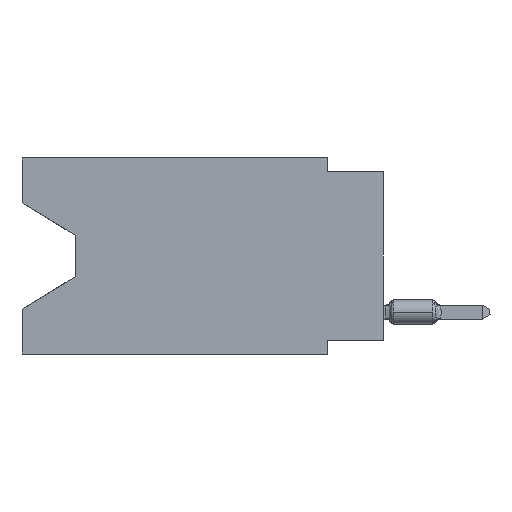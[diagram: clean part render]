
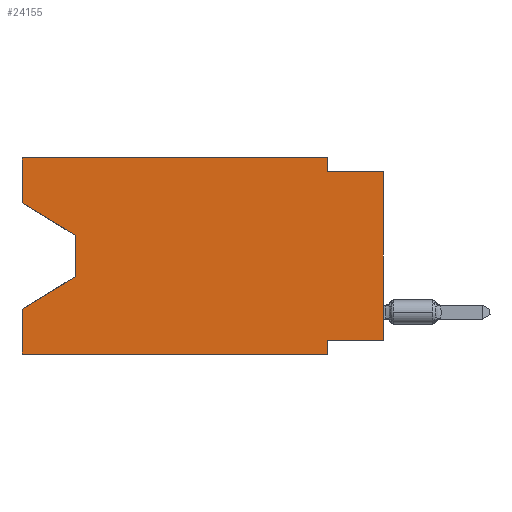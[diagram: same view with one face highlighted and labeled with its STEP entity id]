
A CAD part, left-side view. The second image highlights one B-rep face of the part: STEP entity #24155.
In plain terms, the highlighted planar face has unit normal (-1, 0, 0).
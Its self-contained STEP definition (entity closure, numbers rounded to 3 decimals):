
#120 = VECTOR ( 'NONE', #40571, 1000. ) ;
#173 = CARTESIAN_POINT ( 'NONE',  ( 0., 0., -8.255 ) ) ;
#1086 = LINE ( 'NONE', #61070, #8250 ) ;
#1142 = VERTEX_POINT ( 'NONE', #64276 ) ;
#1245 = VECTOR ( 'NONE', #37471, 1000. ) ;
#1780 = DIRECTION ( 'NONE',  ( 0., -1., 0. ) ) ;
#3478 = DIRECTION ( 'NONE',  ( 0., 0., -1. ) ) ;
#3506 = EDGE_CURVE ( 'NONE', #14370, #38819, #30589, .T. ) ;
#5130 = VERTEX_POINT ( 'NONE', #45987 ) ;
#5617 = ORIENTED_EDGE ( 'NONE', *, *, #63022, .F. ) ;
#6948 = ORIENTED_EDGE ( 'NONE', *, *, #3506, .T. ) ;
#7699 = DIRECTION ( 'NONE',  ( 0., -1., 0. ) ) ;
#8017 = DIRECTION ( 'NONE',  ( 0., 0., 1. ) ) ;
#8250 = VECTOR ( 'NONE', #1780, 1000. ) ;
#8737 = LINE ( 'NONE', #41377, #31765 ) ;
#9317 = CARTESIAN_POINT ( 'NONE',  ( 0., 0., 0. ) ) ;
#9527 = CARTESIAN_POINT ( 'NONE',  ( 0., 13.97, -3.505 ) ) ;
#10179 = VERTEX_POINT ( 'NONE', #19421 ) ;
#10288 = DIRECTION ( 'NONE',  ( 0., 0., 1. ) ) ;
#12784 = EDGE_CURVE ( 'NONE', #42055, #1142, #37810, .T. ) ;
#13929 = EDGE_CURVE ( 'NONE', #19706, #1142, #37487, .T. ) ;
#14370 = VERTEX_POINT ( 'NONE', #43013 ) ;
#14632 = ORIENTED_EDGE ( 'NONE', *, *, #24115, .F. ) ;
#15607 = DIRECTION ( 'NONE',  ( 0., 1., 0. ) ) ;
#15711 = VECTOR ( 'NONE', #38516, 1000. ) ;
#16303 = LINE ( 'NONE', #173, #44985 ) ;
#17675 = DIRECTION ( 'NONE',  ( 0., 0., -1. ) ) ;
#17973 = VERTEX_POINT ( 'NONE', #32679 ) ;
#18152 = ORIENTED_EDGE ( 'NONE', *, *, #36753, .F. ) ;
#19421 = CARTESIAN_POINT ( 'NONE',  ( 0., 16.383, 0. ) ) ;
#19706 = VERTEX_POINT ( 'NONE', #45902 ) ;
#20276 = EDGE_CURVE ( 'NONE', #38819, #17973, #32074, .T. ) ;
#21553 = DIRECTION ( 'NONE',  ( 0., 0.855, -0.519 ) ) ;
#23441 = VECTOR ( 'NONE', #62162, 1000. ) ;
#23731 = VERTEX_POINT ( 'NONE', #44452 ) ;
#24115 = EDGE_CURVE ( 'NONE', #5130, #42055, #16303, .T. ) ;
#24155 = ADVANCED_FACE ( 'NONE', ( #59462 ), #27872, .F. ) ;
#25918 = ORIENTED_EDGE ( 'NONE', *, *, #20276, .T. ) ;
#26005 = ORIENTED_EDGE ( 'NONE', *, *, #45834, .T. ) ;
#26456 = ORIENTED_EDGE ( 'NONE', *, *, #31660, .F. ) ;
#26928 = EDGE_CURVE ( 'NONE', #10179, #68916, #1086, .T. ) ;
#27130 = LINE ( 'NONE', #53101, #38390 ) ;
#27872 = PLANE ( 'NONE',  #48346 ) ;
#28092 = ORIENTED_EDGE ( 'NONE', *, *, #13929, .T. ) ;
#29022 = LINE ( 'NONE', #50795, #67282 ) ;
#29288 = CARTESIAN_POINT ( 'NONE',  ( 0., 16.383, -2.038 ) ) ;
#29448 = LINE ( 'NONE', #45276, #36164 ) ;
#30068 = DIRECTION ( 'NONE',  ( 0., -0.855, -0.519 ) ) ;
#30589 = LINE ( 'NONE', #9527, #23441 ) ;
#30961 = VECTOR ( 'NONE', #21553, 1000. ) ;
#31660 = EDGE_CURVE ( 'NONE', #19706, #17973, #57491, .T. ) ;
#31765 = VECTOR ( 'NONE', #3478, 1000. ) ;
#32074 = LINE ( 'NONE', #59095, #30961 ) ;
#32679 = CARTESIAN_POINT ( 'NONE',  ( 0., 16.383, -6.852 ) ) ;
#34860 = ORIENTED_EDGE ( 'NONE', *, *, #26928, .F. ) ;
#34952 = LINE ( 'NONE', #9317, #120 ) ;
#36164 = VECTOR ( 'NONE', #7699, 1000. ) ;
#36753 = EDGE_CURVE ( 'NONE', #40158, #10179, #27130, .T. ) ;
#37471 = DIRECTION ( 'NONE',  ( 0., 0., -1. ) ) ;
#37487 = LINE ( 'NONE', #54300, #15711 ) ;
#37810 = LINE ( 'NONE', #54629, #1245 ) ;
#38390 = VECTOR ( 'NONE', #10288, 1000. ) ;
#38516 = DIRECTION ( 'NONE',  ( 0., -1., 0. ) ) ;
#38819 = VERTEX_POINT ( 'NONE', #47940 ) ;
#40158 = VERTEX_POINT ( 'NONE', #29288 ) ;
#40571 = DIRECTION ( 'NONE',  ( 0., 0., 1. ) ) ;
#41377 = CARTESIAN_POINT ( 'NONE',  ( 0., 2.54, 0. ) ) ;
#42055 = VERTEX_POINT ( 'NONE', #63720 ) ;
#43013 = CARTESIAN_POINT ( 'NONE',  ( 0., 13.97, -3.505 ) ) ;
#43667 = CARTESIAN_POINT ( 'NONE',  ( 0., 16.383, 0. ) ) ;
#44371 = DIRECTION ( 'NONE',  ( 1., 0., 0. ) ) ;
#44452 = CARTESIAN_POINT ( 'NONE',  ( 0., 0., -0.635 ) ) ;
#44589 = VECTOR ( 'NONE', #8017, 1000. ) ;
#44985 = VECTOR ( 'NONE', #15607, 1000. ) ;
#45276 = CARTESIAN_POINT ( 'NONE',  ( 0., 0., -0.635 ) ) ;
#45834 = EDGE_CURVE ( 'NONE', #40158, #14370, #29022, .T. ) ;
#45902 = CARTESIAN_POINT ( 'NONE',  ( 0., 16.383, -8.89 ) ) ;
#45987 = CARTESIAN_POINT ( 'NONE',  ( 0., 0., -8.255 ) ) ;
#47940 = CARTESIAN_POINT ( 'NONE',  ( 0., 13.97, -5.385 ) ) ;
#48346 = AXIS2_PLACEMENT_3D ( 'NONE', #43667, #44371, #17675 ) ;
#50795 = CARTESIAN_POINT ( 'NONE',  ( 0., 16.383, -2.038 ) ) ;
#53101 = CARTESIAN_POINT ( 'NONE',  ( 0., 16.383, 0. ) ) ;
#54300 = CARTESIAN_POINT ( 'NONE',  ( 0., 16.383, -8.89 ) ) ;
#54629 = CARTESIAN_POINT ( 'NONE',  ( 0., 2.54, -8.89 ) ) ;
#56077 = CARTESIAN_POINT ( 'NONE',  ( 0., 16.383, 0. ) ) ;
#57491 = LINE ( 'NONE', #56077, #44589 ) ;
#58952 = ORIENTED_EDGE ( 'NONE', *, *, #60656, .T. ) ;
#59095 = CARTESIAN_POINT ( 'NONE',  ( 0., 13.97, -5.385 ) ) ;
#59462 = FACE_OUTER_BOUND ( 'NONE', #62516, .T. ) ;
#59767 = VERTEX_POINT ( 'NONE', #63496 ) ;
#60656 = EDGE_CURVE ( 'NONE', #5130, #23731, #34952, .T. ) ;
#61070 = CARTESIAN_POINT ( 'NONE',  ( 0., 16.383, 0. ) ) ;
#62162 = DIRECTION ( 'NONE',  ( 0., 0., -1. ) ) ;
#62223 = ORIENTED_EDGE ( 'NONE', *, *, #69227, .F. ) ;
#62516 = EDGE_LOOP ( 'NONE', ( #26005, #6948, #25918, #26456, #28092, #63371, #14632, #58952, #62223, #5617, #34860, #18152 ) ) ;
#63022 = EDGE_CURVE ( 'NONE', #68916, #59767, #8737, .T. ) ;
#63371 = ORIENTED_EDGE ( 'NONE', *, *, #12784, .F. ) ;
#63496 = CARTESIAN_POINT ( 'NONE',  ( 0., 2.54, -0.635 ) ) ;
#63720 = CARTESIAN_POINT ( 'NONE',  ( 0., 2.54, -8.255 ) ) ;
#64276 = CARTESIAN_POINT ( 'NONE',  ( 0., 2.54, -8.89 ) ) ;
#67282 = VECTOR ( 'NONE', #30068, 1000. ) ;
#67891 = CARTESIAN_POINT ( 'NONE',  ( 0., 2.54, 0. ) ) ;
#68916 = VERTEX_POINT ( 'NONE', #67891 ) ;
#69227 = EDGE_CURVE ( 'NONE', #59767, #23731, #29448, .T. ) ;
